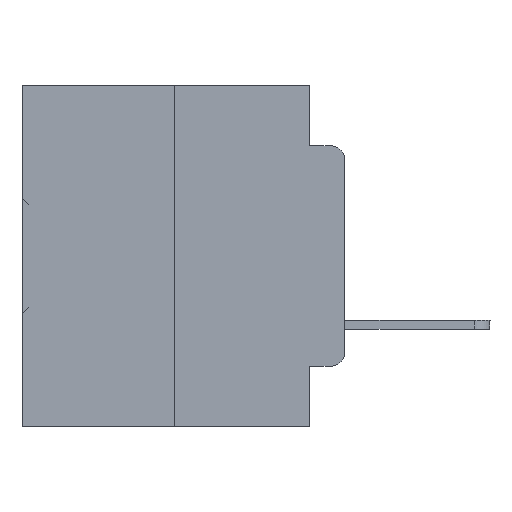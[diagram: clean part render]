
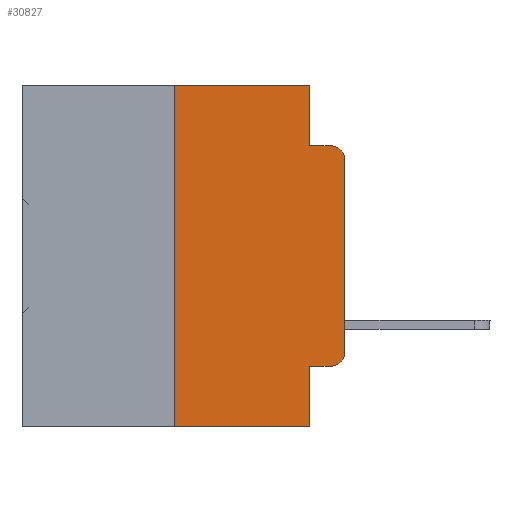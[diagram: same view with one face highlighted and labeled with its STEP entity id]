
A CAD part, left-side view. The second image highlights one B-rep face of the part: STEP entity #30827.
In plain terms, the highlighted planar face has unit normal (-1, 0, 0).
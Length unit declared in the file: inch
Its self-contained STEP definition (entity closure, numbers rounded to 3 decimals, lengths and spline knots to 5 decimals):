
#351 = DIRECTION ( 'NONE',  ( 0., 0., 1. ) ) ;
#821 = VERTEX_POINT ( 'NONE', #6832 ) ;
#893 = CARTESIAN_POINT ( 'NONE',  ( 0., 0.473, 0. ) ) ;
#1548 = EDGE_CURVE ( 'NONE', #5173, #26736, #29100, .T. ) ;
#1574 = PLANE ( 'NONE',  #7442 ) ;
#2865 = VERTEX_POINT ( 'NONE', #14250 ) ;
#2975 = CARTESIAN_POINT ( 'NONE',  ( 0., 0.051, 0. ) ) ;
#4019 = CARTESIAN_POINT ( 'NONE',  ( 0., 0.02, -0.4115 ) ) ;
#4342 = DIRECTION ( 'NONE',  ( 0., 0., -1. ) ) ;
#4903 = VECTOR ( 'NONE', #20553, 39.37008 ) ;
#5173 = VERTEX_POINT ( 'NONE', #18197 ) ;
#5586 = CARTESIAN_POINT ( 'NONE',  ( 0., 0.473, -0.5 ) ) ;
#5852 = AXIS2_PLACEMENT_3D ( 'NONE', #9549, #12313, #21009 ) ;
#6277 = VECTOR ( 'NONE', #20152, 39.37008 ) ;
#6577 = CARTESIAN_POINT ( 'NONE',  ( 0., 0.02, -0.0885 ) ) ;
#6832 = CARTESIAN_POINT ( 'NONE',  ( 0., 0.051, 0. ) ) ;
#7294 = ORIENTED_EDGE ( 'NONE', *, *, #9131, .F. ) ;
#7432 = EDGE_CURVE ( 'NONE', #17711, #32357, #19354, .T. ) ;
#7442 = AXIS2_PLACEMENT_3D ( 'NONE', #10116, #27624, #36096 ) ;
#7688 = CARTESIAN_POINT ( 'NONE',  ( 0., 0.051, -0.4115 ) ) ;
#7990 = ORIENTED_EDGE ( 'NONE', *, *, #33599, .T. ) ;
#8074 = LINE ( 'NONE', #11310, #25620 ) ;
#8326 = VECTOR ( 'NONE', #8346, 39.37008 ) ;
#8346 = DIRECTION ( 'NONE',  ( 0., -1., 0. ) ) ;
#9131 = EDGE_CURVE ( 'NONE', #25628, #9442, #31349, .T. ) ;
#9442 = VERTEX_POINT ( 'NONE', #6577 ) ;
#9549 = CARTESIAN_POINT ( 'NONE',  ( 0., 0.02, -0.1085 ) ) ;
#10116 = CARTESIAN_POINT ( 'NONE',  ( 0., 0.473, 0. ) ) ;
#11197 = LINE ( 'NONE', #2975, #33140 ) ;
#11310 = CARTESIAN_POINT ( 'NONE',  ( 0., 0.051, 0. ) ) ;
#11729 = DIRECTION ( 'NONE',  ( 0., 0., -1. ) ) ;
#11836 = CARTESIAN_POINT ( 'NONE',  ( 0., 0., 0. ) ) ;
#12202 = ORIENTED_EDGE ( 'NONE', *, *, #1548, .T. ) ;
#12313 = DIRECTION ( 'NONE',  ( -1., 0., 0. ) ) ;
#13218 = LINE ( 'NONE', #5586, #8326 ) ;
#14003 = LINE ( 'NONE', #893, #31899 ) ;
#14027 = ORIENTED_EDGE ( 'NONE', *, *, #15675, .F. ) ;
#14250 = CARTESIAN_POINT ( 'NONE',  ( 0., 0.25, -0.5 ) ) ;
#14481 = FACE_OUTER_BOUND ( 'NONE', #16597, .T. ) ;
#14574 = CIRCLE ( 'NONE', #5852, 0.02 ) ;
#15675 = EDGE_CURVE ( 'NONE', #31350, #821, #14003, .T. ) ;
#15996 = VERTEX_POINT ( 'NONE', #21277 ) ;
#16597 = EDGE_LOOP ( 'NONE', ( #12202, #35729, #7294, #29713, #14027, #33686, #34535, #36867, #28452, #7990 ) ) ;
#17092 = DIRECTION ( 'NONE',  ( 0., 0., -1. ) ) ;
#17711 = VERTEX_POINT ( 'NONE', #7688 ) ;
#18197 = CARTESIAN_POINT ( 'NONE',  ( 0., 0., -0.3915 ) ) ;
#19354 = LINE ( 'NONE', #31517, #6277 ) ;
#19779 = CIRCLE ( 'NONE', #31986, 0.02 ) ;
#20152 = DIRECTION ( 'NONE',  ( 0., -1., 0. ) ) ;
#20553 = DIRECTION ( 'NONE',  ( 0., 0., 1. ) ) ;
#21009 = DIRECTION ( 'NONE',  ( 0., 0., -1. ) ) ;
#21277 = CARTESIAN_POINT ( 'NONE',  ( 0., 0.051, -0.5 ) ) ;
#22224 = EDGE_CURVE ( 'NONE', #821, #25628, #8074, .T. ) ;
#24217 = EDGE_CURVE ( 'NONE', #26736, #9442, #14574, .T. ) ;
#25620 = VECTOR ( 'NONE', #17092, 39.37008 ) ;
#25628 = VERTEX_POINT ( 'NONE', #30736 ) ;
#26418 = DIRECTION ( 'NONE',  ( 0., -1., 0. ) ) ;
#26736 = VERTEX_POINT ( 'NONE', #36904 ) ;
#27164 = VECTOR ( 'NONE', #351, 39.37008 ) ;
#27331 = DIRECTION ( 'NONE',  ( -1., 0., 0. ) ) ;
#27624 = DIRECTION ( 'NONE',  ( 1., 0., 0. ) ) ;
#28452 = ORIENTED_EDGE ( 'NONE', *, *, #7432, .T. ) ;
#29100 = LINE ( 'NONE', #11836, #4903 ) ;
#29683 = CARTESIAN_POINT ( 'NONE',  ( 0., 0.051, -0.0885 ) ) ;
#29713 = ORIENTED_EDGE ( 'NONE', *, *, #22224, .F. ) ;
#29934 = DIRECTION ( 'NONE',  ( 0., -1., 0. ) ) ;
#30736 = CARTESIAN_POINT ( 'NONE',  ( 0., 0.051, -0.0885 ) ) ;
#30827 = ADVANCED_FACE ( 'NONE', ( #14481 ), #1574, .F. ) ;
#31349 = LINE ( 'NONE', #29683, #36733 ) ;
#31350 = VERTEX_POINT ( 'NONE', #33466 ) ;
#31517 = CARTESIAN_POINT ( 'NONE',  ( 0., 0.051, -0.4115 ) ) ;
#31635 = LINE ( 'NONE', #36792, #27164 ) ;
#31899 = VECTOR ( 'NONE', #26418, 39.37008 ) ;
#31986 = AXIS2_PLACEMENT_3D ( 'NONE', #35934, #27331, #4342 ) ;
#32357 = VERTEX_POINT ( 'NONE', #4019 ) ;
#33140 = VECTOR ( 'NONE', #11729, 39.37008 ) ;
#33311 = EDGE_CURVE ( 'NONE', #17711, #15996, #11197, .T. ) ;
#33466 = CARTESIAN_POINT ( 'NONE',  ( 0., 0.25, 0. ) ) ;
#33599 = EDGE_CURVE ( 'NONE', #32357, #5173, #19779, .T. ) ;
#33686 = ORIENTED_EDGE ( 'NONE', *, *, #37114, .F. ) ;
#34535 = ORIENTED_EDGE ( 'NONE', *, *, #36966, .T. ) ;
#35729 = ORIENTED_EDGE ( 'NONE', *, *, #24217, .T. ) ;
#35934 = CARTESIAN_POINT ( 'NONE',  ( 0., 0.02, -0.3915 ) ) ;
#36096 = DIRECTION ( 'NONE',  ( 0., 0., -1. ) ) ;
#36733 = VECTOR ( 'NONE', #29934, 39.37008 ) ;
#36792 = CARTESIAN_POINT ( 'NONE',  ( 0., 0.25, 0. ) ) ;
#36867 = ORIENTED_EDGE ( 'NONE', *, *, #33311, .F. ) ;
#36904 = CARTESIAN_POINT ( 'NONE',  ( 0., 0., -0.1085 ) ) ;
#36966 = EDGE_CURVE ( 'NONE', #2865, #15996, #13218, .T. ) ;
#37114 = EDGE_CURVE ( 'NONE', #2865, #31350, #31635, .T. ) ;
